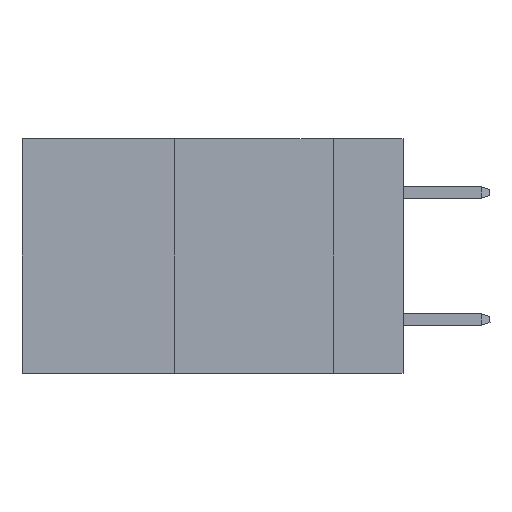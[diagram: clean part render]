
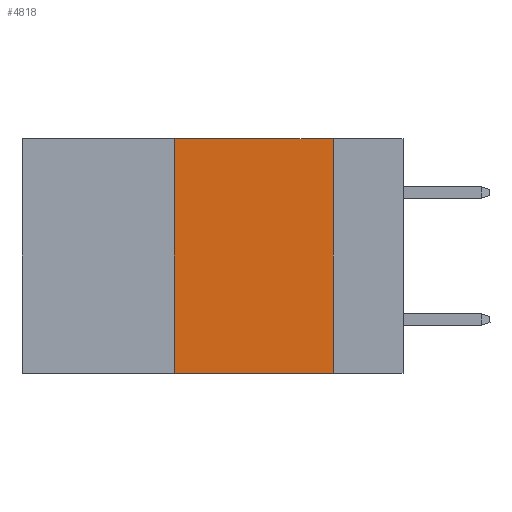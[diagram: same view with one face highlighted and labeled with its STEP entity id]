
A CAD part, left-side view. The second image highlights one B-rep face of the part: STEP entity #4818.
In plain terms, the highlighted planar face has unit normal (-1, 0, 0).
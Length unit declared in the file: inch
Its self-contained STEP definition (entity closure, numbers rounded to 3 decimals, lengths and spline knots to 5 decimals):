
#1046 = DIRECTION ( 'NONE',  ( 0., 0., 1. ) ) ;
#1634 = CARTESIAN_POINT ( 'NONE',  ( 0., 0.36, 0. ) ) ;
#2466 = EDGE_LOOP ( 'NONE', ( #12747, #8083, #11952, #13886 ) ) ;
#3783 = VERTEX_POINT ( 'NONE', #1634 ) ;
#4246 = PLANE ( 'NONE',  #11930 ) ;
#4399 = DIRECTION ( 'NONE',  ( 1., 0., 0. ) ) ;
#4818 = ADVANCED_FACE ( 'NONE', ( #9955 ), #4246, .F. ) ;
#4991 = VERTEX_POINT ( 'NONE', #8520 ) ;
#5453 = DIRECTION ( 'NONE',  ( 0., 0., -1. ) ) ;
#5609 = VERTEX_POINT ( 'NONE', #10955 ) ;
#5972 = EDGE_CURVE ( 'NONE', #4991, #3783, #6668, .T. ) ;
#6665 = CARTESIAN_POINT ( 'NONE',  ( 0., 0.6, 0. ) ) ;
#6668 = LINE ( 'NONE', #11359, #11255 ) ;
#8010 = VERTEX_POINT ( 'NONE', #11680 ) ;
#8083 = ORIENTED_EDGE ( 'NONE', *, *, #10026, .F. ) ;
#8520 = CARTESIAN_POINT ( 'NONE',  ( 0., 0.36, -0.37 ) ) ;
#8868 = DIRECTION ( 'NONE',  ( 0., -1., 0. ) ) ;
#8939 = LINE ( 'NONE', #10198, #13504 ) ;
#9120 = LINE ( 'NONE', #13746, #9647 ) ;
#9647 = VECTOR ( 'NONE', #12539, 39.37008 ) ;
#9955 = FACE_OUTER_BOUND ( 'NONE', #2466, .T. ) ;
#10026 = EDGE_CURVE ( 'NONE', #3783, #5609, #9120, .T. ) ;
#10198 = CARTESIAN_POINT ( 'NONE',  ( 0., 0.6, -0.37 ) ) ;
#10842 = CARTESIAN_POINT ( 'NONE',  ( 0., 0.11, 0. ) ) ;
#10955 = CARTESIAN_POINT ( 'NONE',  ( 0., 0.11, 0. ) ) ;
#11255 = VECTOR ( 'NONE', #1046, 39.37008 ) ;
#11359 = CARTESIAN_POINT ( 'NONE',  ( 0., 0.36, 0. ) ) ;
#11680 = CARTESIAN_POINT ( 'NONE',  ( 0., 0.11, -0.37 ) ) ;
#11930 = AXIS2_PLACEMENT_3D ( 'NONE', #6665, #4399, #5453 ) ;
#11952 = ORIENTED_EDGE ( 'NONE', *, *, #5972, .F. ) ;
#12059 = DIRECTION ( 'NONE',  ( 0., 0., -1. ) ) ;
#12447 = EDGE_CURVE ( 'NONE', #4991, #8010, #8939, .T. ) ;
#12539 = DIRECTION ( 'NONE',  ( 0., -1., 0. ) ) ;
#12747 = ORIENTED_EDGE ( 'NONE', *, *, #12846, .F. ) ;
#12846 = EDGE_CURVE ( 'NONE', #5609, #8010, #12968, .T. ) ;
#12968 = LINE ( 'NONE', #10842, #14474 ) ;
#13504 = VECTOR ( 'NONE', #8868, 39.37008 ) ;
#13746 = CARTESIAN_POINT ( 'NONE',  ( 0., 0.6, 0. ) ) ;
#13886 = ORIENTED_EDGE ( 'NONE', *, *, #12447, .T. ) ;
#14474 = VECTOR ( 'NONE', #12059, 39.37008 ) ;
